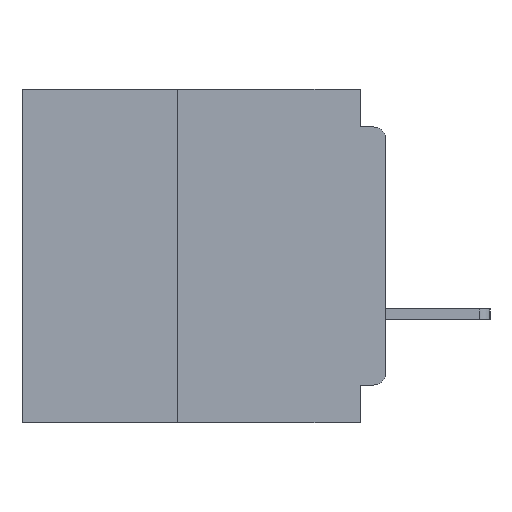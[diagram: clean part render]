
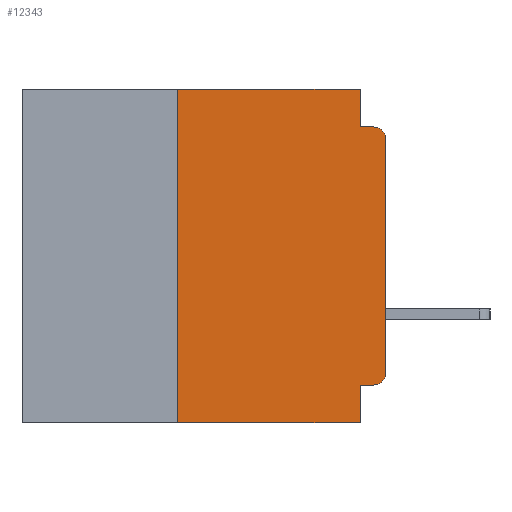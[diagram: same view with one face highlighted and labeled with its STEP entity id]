
A CAD part, left-side view. The second image highlights one B-rep face of the part: STEP entity #12343.
In plain terms, the highlighted planar face has unit normal (-1, 0, 0).
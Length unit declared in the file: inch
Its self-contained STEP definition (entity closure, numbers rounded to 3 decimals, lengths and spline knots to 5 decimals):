
#352 = VERTEX_POINT ( 'NONE', #21020 ) ;
#1061 = CIRCLE ( 'NONE', #33566, 0.015 ) ;
#1213 = CARTESIAN_POINT ( 'NONE',  ( 0., 0.437, 0. ) ) ;
#1533 = LINE ( 'NONE', #38115, #40653 ) ;
#1545 = CARTESIAN_POINT ( 'NONE',  ( 0., 0.015, -0.355 ) ) ;
#2520 = AXIS2_PLACEMENT_3D ( 'NONE', #41344, #18145, #45274 ) ;
#2648 = VECTOR ( 'NONE', #19508, 39.37008 ) ;
#3663 = CARTESIAN_POINT ( 'NONE',  ( 0., 0.25, -0.4 ) ) ;
#4430 = CARTESIAN_POINT ( 'NONE',  ( 0., 0.25, 0. ) ) ;
#5971 = VERTEX_POINT ( 'NONE', #40401 ) ;
#6166 = EDGE_CURVE ( 'NONE', #42771, #49217, #32019, .T. ) ;
#7158 = VERTEX_POINT ( 'NONE', #9894 ) ;
#7647 = CARTESIAN_POINT ( 'NONE',  ( 0., 0.031, -0.4 ) ) ;
#7696 = ORIENTED_EDGE ( 'NONE', *, *, #30234, .F. ) ;
#8869 = ORIENTED_EDGE ( 'NONE', *, *, #40844, .F. ) ;
#9377 = LINE ( 'NONE', #27036, #47110 ) ;
#9894 = CARTESIAN_POINT ( 'NONE',  ( 0., 0.015, -0.045 ) ) ;
#10249 = LINE ( 'NONE', #37581, #29774 ) ;
#10670 = ORIENTED_EDGE ( 'NONE', *, *, #14300, .T. ) ;
#11928 = EDGE_CURVE ( 'NONE', #35109, #22079, #9377, .T. ) ;
#12343 = ADVANCED_FACE ( 'NONE', ( #17346 ), #40338, .F. ) ;
#12472 = EDGE_LOOP ( 'NONE', ( #32625, #10670, #7696, #16423, #8869, #15783, #41541, #25775, #23166, #18930 ) ) ;
#13632 = CARTESIAN_POINT ( 'NONE',  ( 0., 0., -0.34 ) ) ;
#13987 = CARTESIAN_POINT ( 'NONE',  ( 0., 0.015, -0.34 ) ) ;
#14300 = EDGE_CURVE ( 'NONE', #352, #7158, #37116, .T. ) ;
#14390 = DIRECTION ( 'NONE',  ( 0., -1., 0. ) ) ;
#15783 = ORIENTED_EDGE ( 'NONE', *, *, #11928, .F. ) ;
#15855 = LINE ( 'NONE', #47430, #35244 ) ;
#16423 = ORIENTED_EDGE ( 'NONE', *, *, #6166, .F. ) ;
#17346 = FACE_OUTER_BOUND ( 'NONE', #12472, .T. ) ;
#17863 = DIRECTION ( 'NONE',  ( 0., 0., -1. ) ) ;
#18052 = EDGE_CURVE ( 'NONE', #22248, #352, #29932, .T. ) ;
#18145 = DIRECTION ( 'NONE',  ( -1., 0., 0. ) ) ;
#18930 = ORIENTED_EDGE ( 'NONE', *, *, #39206, .T. ) ;
#19508 = DIRECTION ( 'NONE',  ( 0., 0., -1. ) ) ;
#20631 = CARTESIAN_POINT ( 'NONE',  ( 0., 0.031, -0.045 ) ) ;
#21020 = CARTESIAN_POINT ( 'NONE',  ( 0., 0., -0.06 ) ) ;
#21056 = DIRECTION ( 'NONE',  ( 0., 0., -1. ) ) ;
#21722 = VECTOR ( 'NONE', #26417, 39.37008 ) ;
#22019 = VECTOR ( 'NONE', #47558, 39.37008 ) ;
#22079 = VERTEX_POINT ( 'NONE', #4430 ) ;
#22248 = VERTEX_POINT ( 'NONE', #13632 ) ;
#23166 = ORIENTED_EDGE ( 'NONE', *, *, #49152, .F. ) ;
#23597 = LINE ( 'NONE', #7647, #2648 ) ;
#25775 = ORIENTED_EDGE ( 'NONE', *, *, #42698, .F. ) ;
#26417 = DIRECTION ( 'NONE',  ( 0., 0., -1. ) ) ;
#27036 = CARTESIAN_POINT ( 'NONE',  ( 0., 0.25, -0.4 ) ) ;
#28162 = DIRECTION ( 'NONE',  ( 0., 1., 0. ) ) ;
#28738 = VECTOR ( 'NONE', #34744, 39.37008 ) ;
#29774 = VECTOR ( 'NONE', #14390, 39.37008 ) ;
#29932 = LINE ( 'NONE', #30877, #28738 ) ;
#30234 = EDGE_CURVE ( 'NONE', #49217, #7158, #42610, .T. ) ;
#30874 = DIRECTION ( 'NONE',  ( 0., 0., 1. ) ) ;
#30877 = CARTESIAN_POINT ( 'NONE',  ( 0., 0., 0. ) ) ;
#31578 = EDGE_CURVE ( 'NONE', #35109, #42987, #10249, .T. ) ;
#32019 = LINE ( 'NONE', #37833, #21722 ) ;
#32625 = ORIENTED_EDGE ( 'NONE', *, *, #18052, .T. ) ;
#33566 = AXIS2_PLACEMENT_3D ( 'NONE', #13987, #41063, #17863 ) ;
#34744 = DIRECTION ( 'NONE',  ( 0., 0., 1. ) ) ;
#35109 = VERTEX_POINT ( 'NONE', #3663 ) ;
#35244 = VECTOR ( 'NONE', #28162, 39.37008 ) ;
#37116 = CIRCLE ( 'NONE', #2520, 0.015 ) ;
#37581 = CARTESIAN_POINT ( 'NONE',  ( 0., 0.437, -0.4 ) ) ;
#37833 = CARTESIAN_POINT ( 'NONE',  ( 0., 0.031, 0. ) ) ;
#38115 = CARTESIAN_POINT ( 'NONE',  ( 0., 0.437, 0. ) ) ;
#39206 = EDGE_CURVE ( 'NONE', #48411, #22248, #1061, .T. ) ;
#39295 = CARTESIAN_POINT ( 'NONE',  ( 0., 0.031, 0. ) ) ;
#40338 = PLANE ( 'NONE',  #42387 ) ;
#40401 = CARTESIAN_POINT ( 'NONE',  ( 0., 0.031, -0.355 ) ) ;
#40636 = CARTESIAN_POINT ( 'NONE',  ( 0., 0.031, -0.4 ) ) ;
#40653 = VECTOR ( 'NONE', #42004, 39.37008 ) ;
#40844 = EDGE_CURVE ( 'NONE', #22079, #42771, #1533, .T. ) ;
#41063 = DIRECTION ( 'NONE',  ( -1., 0., 0. ) ) ;
#41344 = CARTESIAN_POINT ( 'NONE',  ( 0., 0.015, -0.06 ) ) ;
#41541 = ORIENTED_EDGE ( 'NONE', *, *, #31578, .T. ) ;
#42004 = DIRECTION ( 'NONE',  ( 0., -1., 0. ) ) ;
#42387 = AXIS2_PLACEMENT_3D ( 'NONE', #1213, #44266, #21056 ) ;
#42610 = LINE ( 'NONE', #43647, #22019 ) ;
#42698 = EDGE_CURVE ( 'NONE', #5971, #42987, #23597, .T. ) ;
#42771 = VERTEX_POINT ( 'NONE', #39295 ) ;
#42987 = VERTEX_POINT ( 'NONE', #40636 ) ;
#43647 = CARTESIAN_POINT ( 'NONE',  ( 0., 0., -0.045 ) ) ;
#44266 = DIRECTION ( 'NONE',  ( 1., 0., 0. ) ) ;
#45274 = DIRECTION ( 'NONE',  ( 0., 0., -1. ) ) ;
#47110 = VECTOR ( 'NONE', #30874, 39.37008 ) ;
#47430 = CARTESIAN_POINT ( 'NONE',  ( 0., 0., -0.355 ) ) ;
#47558 = DIRECTION ( 'NONE',  ( 0., -1., 0. ) ) ;
#48411 = VERTEX_POINT ( 'NONE', #1545 ) ;
#49152 = EDGE_CURVE ( 'NONE', #48411, #5971, #15855, .T. ) ;
#49217 = VERTEX_POINT ( 'NONE', #20631 ) ;
